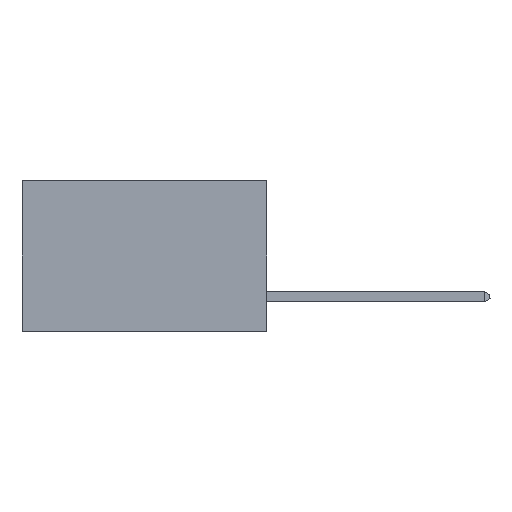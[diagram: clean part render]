
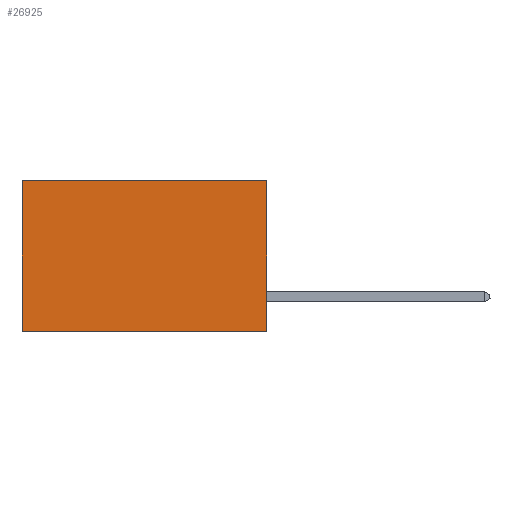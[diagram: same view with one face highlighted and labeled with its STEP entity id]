
A CAD part, left-side view. The second image highlights one B-rep face of the part: STEP entity #26925.
In plain terms, the highlighted planar face has unit normal (-1, 0, 0).
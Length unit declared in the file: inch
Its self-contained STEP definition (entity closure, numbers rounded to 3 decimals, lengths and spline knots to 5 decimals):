
#401 = CARTESIAN_POINT ( 'NONE',  ( 0.2875, 0., 0. ) ) ;
#993 = VECTOR ( 'NONE', #31133, 39.37008 ) ;
#1555 = CARTESIAN_POINT ( 'NONE',  ( 0.2875, 0.6, -0.37 ) ) ;
#2042 = LINE ( 'NONE', #21702, #993 ) ;
#4385 = EDGE_CURVE ( 'NONE', #5727, #7180, #5307, .T. ) ;
#5307 = LINE ( 'NONE', #39835, #36198 ) ;
#5727 = VERTEX_POINT ( 'NONE', #15624 ) ;
#6199 = CARTESIAN_POINT ( 'NONE',  ( 0.2875, 0., -0.37 ) ) ;
#6243 = ORIENTED_EDGE ( 'NONE', *, *, #12900, .T. ) ;
#6502 = VERTEX_POINT ( 'NONE', #13381 ) ;
#6763 = DIRECTION ( 'NONE',  ( 0., 0., -1. ) ) ;
#7180 = VERTEX_POINT ( 'NONE', #20123 ) ;
#12595 = EDGE_LOOP ( 'NONE', ( #32433, #31239, #38204, #6243 ) ) ;
#12900 = EDGE_CURVE ( 'NONE', #5727, #6502, #2042, .T. ) ;
#13381 = CARTESIAN_POINT ( 'NONE',  ( 0.2875, 0.6, 0. ) ) ;
#13741 = VECTOR ( 'NONE', #35027, 39.37008 ) ;
#14956 = AXIS2_PLACEMENT_3D ( 'NONE', #401, #22706, #6763 ) ;
#15624 = CARTESIAN_POINT ( 'NONE',  ( 0.2875, 0., 0. ) ) ;
#19756 = PLANE ( 'NONE',  #14956 ) ;
#20123 = CARTESIAN_POINT ( 'NONE',  ( 0.2875, 0., -0.37 ) ) ;
#20614 = DIRECTION ( 'NONE',  ( 0., 0., -1. ) ) ;
#21702 = CARTESIAN_POINT ( 'NONE',  ( 0.2875, 0., 0. ) ) ;
#22706 = DIRECTION ( 'NONE',  ( 1., 0., 0. ) ) ;
#24973 = EDGE_CURVE ( 'NONE', #7180, #32987, #37243, .T. ) ;
#26925 = ADVANCED_FACE ( 'NONE', ( #31616 ), #19756, .F. ) ;
#31133 = DIRECTION ( 'NONE',  ( 0., 1., 0. ) ) ;
#31239 = ORIENTED_EDGE ( 'NONE', *, *, #24973, .F. ) ;
#31412 = VECTOR ( 'NONE', #37781, 39.37008 ) ;
#31616 = FACE_OUTER_BOUND ( 'NONE', #12595, .T. ) ;
#32433 = ORIENTED_EDGE ( 'NONE', *, *, #38704, .T. ) ;
#32856 = LINE ( 'NONE', #36269, #31412 ) ;
#32987 = VERTEX_POINT ( 'NONE', #1555 ) ;
#35027 = DIRECTION ( 'NONE',  ( 0., 1., 0. ) ) ;
#36198 = VECTOR ( 'NONE', #20614, 39.37008 ) ;
#36269 = CARTESIAN_POINT ( 'NONE',  ( 0.2875, 0.6, 0. ) ) ;
#37243 = LINE ( 'NONE', #6199, #13741 ) ;
#37781 = DIRECTION ( 'NONE',  ( 0., 0., -1. ) ) ;
#38204 = ORIENTED_EDGE ( 'NONE', *, *, #4385, .F. ) ;
#38704 = EDGE_CURVE ( 'NONE', #6502, #32987, #32856, .T. ) ;
#39835 = CARTESIAN_POINT ( 'NONE',  ( 0.2875, 0., 0. ) ) ;
